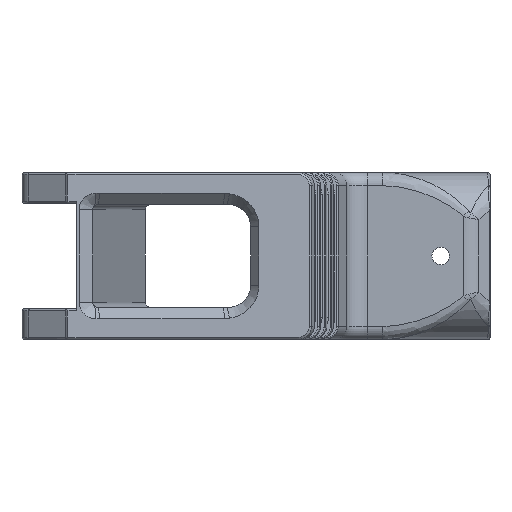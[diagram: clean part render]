
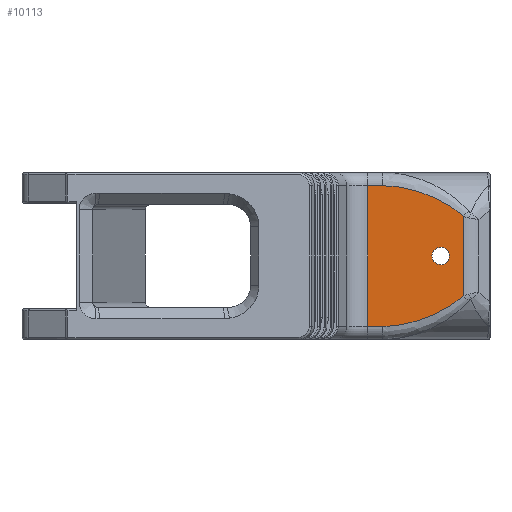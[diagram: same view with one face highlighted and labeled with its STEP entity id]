
A CAD part, front view. The second image highlights one B-rep face of the part: STEP entity #10113.
In plain terms, the highlighted planar face has unit normal (0, -1, 0).
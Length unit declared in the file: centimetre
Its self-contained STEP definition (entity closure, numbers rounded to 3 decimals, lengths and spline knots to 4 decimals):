
#299=CIRCLE($,#10936,0.2);
#741=FACE_BOUND($,#1998,.T.);
#860=PLANE($,#10935);
#1354=FACE_OUTER_BOUND($,#1997,.T.);
#1997=EDGE_LOOP($,(#8583,#8584,#8585,#8586,#8587,#8588));
#1998=EDGE_LOOP($,(#8589));
#2744=LINE($,#19931,#3504);
#2745=LINE($,#19942,#3505);
#2746=LINE($,#19944,#3506);
#2747=LINE($,#19946,#3507);
#3504=VECTOR($,#12979,1.8036);
#3505=VECTOR($,#12982,0.3447);
#3506=VECTOR($,#12983,3.2);
#3507=VECTOR($,#12984,0.3447);
#3983=B_SPLINE_CURVE_WITH_KNOTS($,3,(#19934,#19935,#19936,#19937,#19938,
#19939,#19940),.UNSPECIFIED.,.F.,.F.,(4,1,1,1,4),(0.,
0.5714,1.1428,1.7141,1.9998),
 .UNSPECIFIED.);
#3984=B_SPLINE_CURVE_WITH_KNOTS($,3,(#19947,#19948,#19949,#19950,#19951,
#19952,#19953),.UNSPECIFIED.,.F.,.F.,(4,1,1,1,4),(3.8425,4.1282,
4.6996,5.271,5.8424),.UNSPECIFIED.);
#4741=VERTEX_POINT($,#19838);
#4743=VERTEX_POINT($,#19893);
#4744=VERTEX_POINT($,#19933);
#4745=VERTEX_POINT($,#19941);
#4746=VERTEX_POINT($,#19943);
#4747=VERTEX_POINT($,#19945);
#4748=VERTEX_POINT($,#19954);
#6075=EDGE_CURVE($,#4743,#4741,#2744,.T.);
#6076=EDGE_CURVE($,#4744,#4743,#3983,.T.);
#6077=EDGE_CURVE($,#4745,#4744,#2745,.T.);
#6078=EDGE_CURVE($,#4745,#4746,#2746,.T.);
#6079=EDGE_CURVE($,#4747,#4746,#2747,.T.);
#6080=EDGE_CURVE($,#4741,#4747,#3984,.T.);
#6081=EDGE_CURVE($,#4748,#4748,#299,.T.);
#8583=ORIENTED_EDGE($,*,*,#6075,.F.);
#8584=ORIENTED_EDGE($,*,*,#6076,.F.);
#8585=ORIENTED_EDGE($,*,*,#6077,.F.);
#8586=ORIENTED_EDGE($,*,*,#6078,.T.);
#8587=ORIENTED_EDGE($,*,*,#6079,.F.);
#8588=ORIENTED_EDGE($,*,*,#6080,.F.);
#8589=ORIENTED_EDGE($,*,*,#6081,.F.);
#10113=ADVANCED_FACE($,(#1354,#741),#860,.T.);
#10935=AXIS2_PLACEMENT_3D($,#19932,#12980,#12981);
#10936=AXIS2_PLACEMENT_3D($,#19955,#12985,#12986);
#12979=DIRECTION($,(0.,0.,-1.));
#12980=DIRECTION('center_axis',(0.,-1.,0.));
#12981=DIRECTION('ref_axis',(0.,0.,-1.));
#12982=DIRECTION($,(1.,0.,0.));
#12983=DIRECTION($,(0.,0.,-1.));
#12984=DIRECTION($,(-1.,0.,0.));
#12985=DIRECTION('center_axis',(0.,-1.,0.));
#12986=DIRECTION('ref_axis',(1.,0.,0.));
#19838=CARTESIAN_POINT('',(0.5606,-2.5877,-10.4018));
#19893=CARTESIAN_POINT('',(0.5606,-2.5877,-8.5982));
#19931=CARTESIAN_POINT($,(0.5606,-2.5877,-9.4897));
#19932=CARTESIAN_POINT('Origin',(0.6464,-2.5877,-9.5));
#19933=CARTESIAN_POINT('',(-1.2702,-2.5877,-7.9));
#19934=CARTESIAN_POINT('Ctrl Pts',(-1.2702,-2.5877,
-7.9));
#19935=CARTESIAN_POINT('Ctrl Pts',(-1.0797,-2.5877,
-7.9));
#19936=CARTESIAN_POINT('Ctrl Pts',(-0.6992,-2.5877,
-7.9476));
#19937=CARTESIAN_POINT('Ctrl Pts',(-0.1559,-2.5877,
-8.1305));
#19938=CARTESIAN_POINT('Ctrl Pts',(0.2634,-2.5877,
-8.3585));
#19939=CARTESIAN_POINT('Ctrl Pts',(0.4905,-2.5877,
-8.5339));
#19940=CARTESIAN_POINT('Ctrl Pts',(0.5606,-2.5877,
-8.5982));
#19941=CARTESIAN_POINT('',(-1.6149,-2.5877,-7.9));
#19942=CARTESIAN_POINT($,(-1.9118,-2.5877,-7.9));
#19943=CARTESIAN_POINT('',(-1.6149,-2.5877,-11.1));
#19944=CARTESIAN_POINT($,(-1.6149,-2.5877,-9.5));
#19945=CARTESIAN_POINT('',(-1.2702,-2.5877,-11.1));
#19946=CARTESIAN_POINT($,(-1.9118,-2.5877,-11.1));
#19947=CARTESIAN_POINT('Ctrl Pts',(0.5606,-2.5877,
-10.4018));
#19948=CARTESIAN_POINT('Ctrl Pts',(0.4905,-2.5877,
-10.4661));
#19949=CARTESIAN_POINT('Ctrl Pts',(0.2634,-2.5877,
-10.6415));
#19950=CARTESIAN_POINT('Ctrl Pts',(-0.1559,-2.5877,
-10.8695));
#19951=CARTESIAN_POINT('Ctrl Pts',(-0.6992,-2.5877,
-11.0524));
#19952=CARTESIAN_POINT('Ctrl Pts',(-1.0797,-2.5877,
-11.1));
#19953=CARTESIAN_POINT('Ctrl Pts',(-1.2702,-2.5877,-11.1));
#19954=CARTESIAN_POINT('',(-0.1536,-2.5877,-9.5));
#19955=CARTESIAN_POINT('Origin',(0.0464,-2.5877,-9.5));
